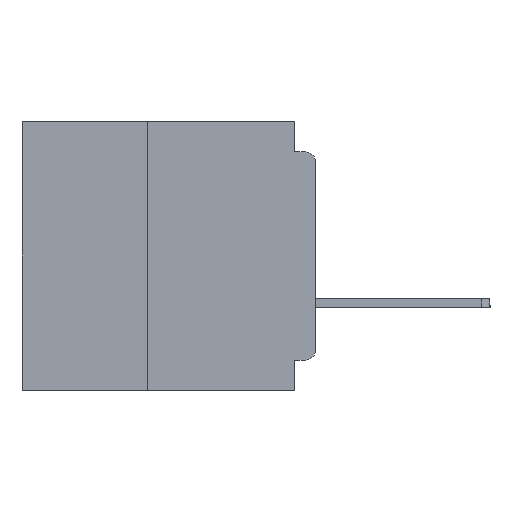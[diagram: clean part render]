
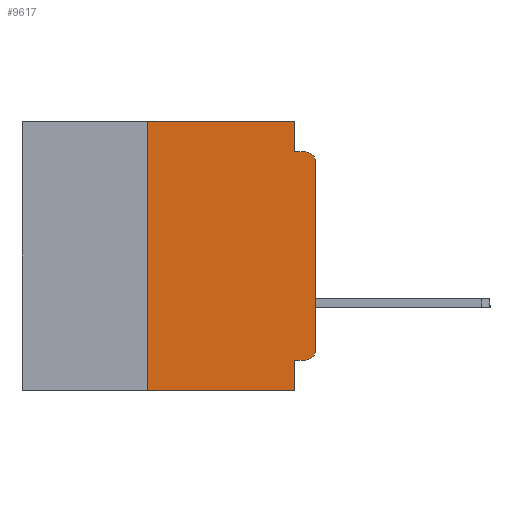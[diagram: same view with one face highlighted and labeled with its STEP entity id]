
A CAD part, left-side view. The second image highlights one B-rep face of the part: STEP entity #9617.
In plain terms, the highlighted planar face has unit normal (-1, 0, 0).
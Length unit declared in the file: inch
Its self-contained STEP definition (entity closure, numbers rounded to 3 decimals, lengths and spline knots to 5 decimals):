
#131 = VERTEX_POINT ( 'NONE', #18948 ) ;
#733 = DIRECTION ( 'NONE',  ( 0., -1., 0. ) ) ;
#966 = VERTEX_POINT ( 'NONE', #34021 ) ;
#1271 = ORIENTED_EDGE ( 'NONE', *, *, #3047, .F. ) ;
#1610 = CIRCLE ( 'NONE', #37066, 0.015 ) ;
#2539 = CARTESIAN_POINT ( 'NONE',  ( 0., 0., -0.06 ) ) ;
#3047 = EDGE_CURVE ( 'NONE', #55584, #25663, #5122, .T. ) ;
#3281 = VERTEX_POINT ( 'NONE', #5408 ) ;
#3661 = VECTOR ( 'NONE', #29733, 39.37008 ) ;
#4515 = CARTESIAN_POINT ( 'NONE',  ( 0., 0., -0.355 ) ) ;
#4523 = EDGE_CURVE ( 'NONE', #57228, #3281, #45632, .T. ) ;
#5005 = LINE ( 'NONE', #54321, #19130 ) ;
#5122 = LINE ( 'NONE', #54340, #54102 ) ;
#5408 = CARTESIAN_POINT ( 'NONE',  ( 0., 0.015, -0.045 ) ) ;
#5521 = CARTESIAN_POINT ( 'NONE',  ( 0., 0.437, 0. ) ) ;
#9517 = EDGE_CURVE ( 'NONE', #19719, #131, #43473, .T. ) ;
#9617 = ADVANCED_FACE ( 'NONE', ( #35725 ), #22776, .F. ) ;
#10464 = VERTEX_POINT ( 'NONE', #24952 ) ;
#12537 = CARTESIAN_POINT ( 'NONE',  ( 0., 0.031, 0. ) ) ;
#12746 = ORIENTED_EDGE ( 'NONE', *, *, #47183, .F. ) ;
#14367 = VERTEX_POINT ( 'NONE', #55097 ) ;
#16272 = LINE ( 'NONE', #58067, #3661 ) ;
#16409 = LINE ( 'NONE', #5521, #40232 ) ;
#18183 = CARTESIAN_POINT ( 'NONE',  ( 0., 0.437, 0. ) ) ;
#18248 = VERTEX_POINT ( 'NONE', #49978 ) ;
#18263 = AXIS2_PLACEMENT_3D ( 'NONE', #18183, #22987, #56087 ) ;
#18948 = CARTESIAN_POINT ( 'NONE',  ( 0., 0.031, -0.045 ) ) ;
#19130 = VECTOR ( 'NONE', #54515, 39.37008 ) ;
#19626 = EDGE_LOOP ( 'NONE', ( #59228, #50913, #33307, #35679, #12746, #1271, #22728, #25490, #46239, #55923 ) ) ;
#19719 = VERTEX_POINT ( 'NONE', #12537 ) ;
#20318 = EDGE_CURVE ( 'NONE', #10464, #966, #1610, .T. ) ;
#21831 = DIRECTION ( 'NONE',  ( -1., 0., 0. ) ) ;
#22728 = ORIENTED_EDGE ( 'NONE', *, *, #53302, .T. ) ;
#22776 = PLANE ( 'NONE',  #18263 ) ;
#22987 = DIRECTION ( 'NONE',  ( 1., 0., 0. ) ) ;
#23062 = VECTOR ( 'NONE', #26775, 39.37008 ) ;
#23666 = DIRECTION ( 'NONE',  ( 0., 1., 0. ) ) ;
#24342 = LINE ( 'NONE', #4515, #35484 ) ;
#24952 = CARTESIAN_POINT ( 'NONE',  ( 0., 0.015, -0.355 ) ) ;
#25490 = ORIENTED_EDGE ( 'NONE', *, *, #41987, .F. ) ;
#25663 = VERTEX_POINT ( 'NONE', #44509 ) ;
#26775 = DIRECTION ( 'NONE',  ( 0., -1., 0. ) ) ;
#27559 = EDGE_CURVE ( 'NONE', #966, #57228, #34574, .T. ) ;
#27873 = VECTOR ( 'NONE', #50555, 39.37008 ) ;
#29733 = DIRECTION ( 'NONE',  ( 0., -1., 0. ) ) ;
#31554 = CARTESIAN_POINT ( 'NONE',  ( 0., 0.437, -0.4 ) ) ;
#33307 = ORIENTED_EDGE ( 'NONE', *, *, #53625, .F. ) ;
#34021 = CARTESIAN_POINT ( 'NONE',  ( 0., 0., -0.34 ) ) ;
#34574 = LINE ( 'NONE', #44488, #58200 ) ;
#34994 = DIRECTION ( 'NONE',  ( 0., 0., 1. ) ) ;
#35484 = VECTOR ( 'NONE', #23666, 39.37008 ) ;
#35679 = ORIENTED_EDGE ( 'NONE', *, *, #9517, .F. ) ;
#35725 = FACE_OUTER_BOUND ( 'NONE', #19626, .T. ) ;
#36533 = EDGE_CURVE ( 'NONE', #10464, #18248, #24342, .T. ) ;
#37066 = AXIS2_PLACEMENT_3D ( 'NONE', #50227, #21831, #54980 ) ;
#40232 = VECTOR ( 'NONE', #733, 39.37008 ) ;
#41987 = EDGE_CURVE ( 'NONE', #18248, #14367, #5005, .T. ) ;
#43473 = LINE ( 'NONE', #55294, #27873 ) ;
#44488 = CARTESIAN_POINT ( 'NONE',  ( 0., 0., 0. ) ) ;
#44509 = CARTESIAN_POINT ( 'NONE',  ( 0., 0.25, 0. ) ) ;
#45632 = CIRCLE ( 'NONE', #58813, 0.015 ) ;
#46239 = ORIENTED_EDGE ( 'NONE', *, *, #36533, .F. ) ;
#47183 = EDGE_CURVE ( 'NONE', #25663, #19719, #16409, .T. ) ;
#49092 = DIRECTION ( 'NONE',  ( 0., 0., -1. ) ) ;
#49292 = DIRECTION ( 'NONE',  ( -1., 0., 0. ) ) ;
#49409 = CARTESIAN_POINT ( 'NONE',  ( 0., 0.015, -0.06 ) ) ;
#49978 = CARTESIAN_POINT ( 'NONE',  ( 0., 0.031, -0.355 ) ) ;
#50227 = CARTESIAN_POINT ( 'NONE',  ( 0., 0.015, -0.34 ) ) ;
#50555 = DIRECTION ( 'NONE',  ( 0., 0., -1. ) ) ;
#50913 = ORIENTED_EDGE ( 'NONE', *, *, #4523, .T. ) ;
#53302 = EDGE_CURVE ( 'NONE', #55584, #14367, #60744, .T. ) ;
#53625 = EDGE_CURVE ( 'NONE', #131, #3281, #16272, .T. ) ;
#54102 = VECTOR ( 'NONE', #54381, 39.37008 ) ;
#54321 = CARTESIAN_POINT ( 'NONE',  ( 0., 0.031, -0.4 ) ) ;
#54340 = CARTESIAN_POINT ( 'NONE',  ( 0., 0.25, -0.4 ) ) ;
#54381 = DIRECTION ( 'NONE',  ( 0., 0., 1. ) ) ;
#54515 = DIRECTION ( 'NONE',  ( 0., 0., -1. ) ) ;
#54980 = DIRECTION ( 'NONE',  ( 0., 0., -1. ) ) ;
#55097 = CARTESIAN_POINT ( 'NONE',  ( 0., 0.031, -0.4 ) ) ;
#55294 = CARTESIAN_POINT ( 'NONE',  ( 0., 0.031, 0. ) ) ;
#55584 = VERTEX_POINT ( 'NONE', #59878 ) ;
#55923 = ORIENTED_EDGE ( 'NONE', *, *, #20318, .T. ) ;
#56087 = DIRECTION ( 'NONE',  ( 0., 0., -1. ) ) ;
#57228 = VERTEX_POINT ( 'NONE', #2539 ) ;
#58067 = CARTESIAN_POINT ( 'NONE',  ( 0., 0., -0.045 ) ) ;
#58200 = VECTOR ( 'NONE', #34994, 39.37008 ) ;
#58813 = AXIS2_PLACEMENT_3D ( 'NONE', #49409, #49292, #49092 ) ;
#59228 = ORIENTED_EDGE ( 'NONE', *, *, #27559, .T. ) ;
#59878 = CARTESIAN_POINT ( 'NONE',  ( 0., 0.25, -0.4 ) ) ;
#60744 = LINE ( 'NONE', #31554, #23062 ) ;
